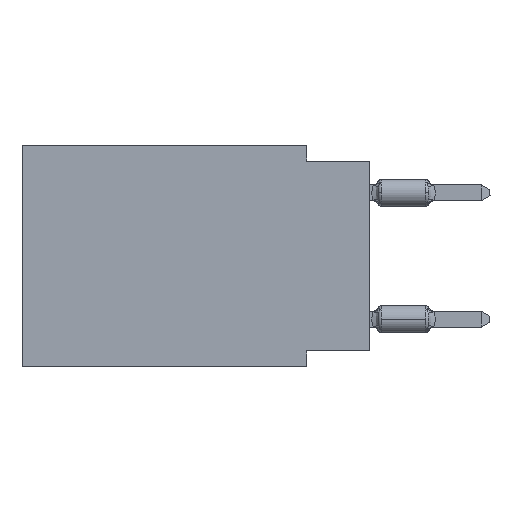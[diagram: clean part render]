
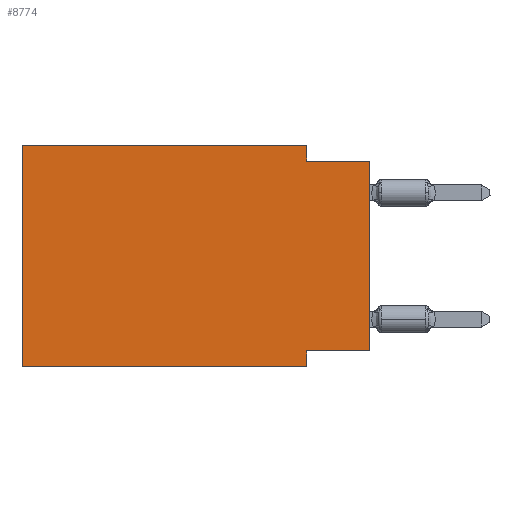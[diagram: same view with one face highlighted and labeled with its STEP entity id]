
A CAD part, left-side view. The second image highlights one B-rep face of the part: STEP entity #8774.
In plain terms, the highlighted planar face has unit normal (-1, 0, 0).
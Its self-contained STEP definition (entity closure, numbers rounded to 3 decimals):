
#552 = CARTESIAN_POINT ( 'NONE',  ( 0., 13.97, 0. ) ) ;
#872 = VECTOR ( 'NONE', #2977, 1000. ) ;
#1038 = ORIENTED_EDGE ( 'NONE', *, *, #6615, .T. ) ;
#1206 = CARTESIAN_POINT ( 'NONE',  ( 0., 2.54, -8.89 ) ) ;
#1652 = PLANE ( 'NONE',  #12553 ) ;
#1987 = ORIENTED_EDGE ( 'NONE', *, *, #8923, .F. ) ;
#2245 = CARTESIAN_POINT ( 'NONE',  ( 0., 2.54, -0.635 ) ) ;
#2977 = DIRECTION ( 'NONE',  ( 0., 0., -1. ) ) ;
#3429 = ORIENTED_EDGE ( 'NONE', *, *, #5360, .F. ) ;
#3430 = DIRECTION ( 'NONE',  ( 0., -1., 0. ) ) ;
#3570 = DIRECTION ( 'NONE',  ( 0., 0., -1. ) ) ;
#4036 = CARTESIAN_POINT ( 'NONE',  ( 0., 2.54, -8.255 ) ) ;
#4069 = CARTESIAN_POINT ( 'NONE',  ( 0., 2.54, 0. ) ) ;
#4144 = CARTESIAN_POINT ( 'NONE',  ( 0., 0., -8.255 ) ) ;
#4422 = VECTOR ( 'NONE', #27921, 1000. ) ;
#5103 = CARTESIAN_POINT ( 'NONE',  ( 0., 0., -0.635 ) ) ;
#5360 = EDGE_CURVE ( 'NONE', #18865, #16449, #18100, .T. ) ;
#5438 = CARTESIAN_POINT ( 'NONE',  ( 0., 2.54, 0. ) ) ;
#6615 = EDGE_CURVE ( 'NONE', #22072, #22114, #7286, .T. ) ;
#6619 = LINE ( 'NONE', #4144, #24721 ) ;
#6638 = EDGE_CURVE ( 'NONE', #8939, #22114, #17953, .T. ) ;
#7006 = DIRECTION ( 'NONE',  ( 0., -1., 0. ) ) ;
#7286 = LINE ( 'NONE', #16025, #12534 ) ;
#7339 = VECTOR ( 'NONE', #15163, 1000. ) ;
#7668 = LINE ( 'NONE', #12634, #13821 ) ;
#8774 = ADVANCED_FACE ( 'NONE', ( #25801 ), #1652, .F. ) ;
#8918 = ORIENTED_EDGE ( 'NONE', *, *, #18597, .F. ) ;
#8923 = EDGE_CURVE ( 'NONE', #22072, #18111, #6619, .T. ) ;
#8939 = VERTEX_POINT ( 'NONE', #2245 ) ;
#9040 = DIRECTION ( 'NONE',  ( 0., 0., 1. ) ) ;
#9163 = VERTEX_POINT ( 'NONE', #5438 ) ;
#9680 = VECTOR ( 'NONE', #18386, 1000. ) ;
#10164 = CARTESIAN_POINT ( 'NONE',  ( 0., 0., -0.635 ) ) ;
#10265 = CARTESIAN_POINT ( 'NONE',  ( 0., 2.54, -8.89 ) ) ;
#10452 = CARTESIAN_POINT ( 'NONE',  ( 0., 0., -8.255 ) ) ;
#11527 = CARTESIAN_POINT ( 'NONE',  ( 0., 13.97, 0. ) ) ;
#12534 = VECTOR ( 'NONE', #9040, 1000. ) ;
#12553 = AXIS2_PLACEMENT_3D ( 'NONE', #23609, #21689, #3570 ) ;
#12634 = CARTESIAN_POINT ( 'NONE',  ( 0., 13.97, 0. ) ) ;
#13142 = EDGE_CURVE ( 'NONE', #18865, #27840, #14449, .T. ) ;
#13821 = VECTOR ( 'NONE', #3430, 1000. ) ;
#14002 = ORIENTED_EDGE ( 'NONE', *, *, #16421, .F. ) ;
#14449 = LINE ( 'NONE', #26012, #4422 ) ;
#15028 = LINE ( 'NONE', #4069, #7339 ) ;
#15163 = DIRECTION ( 'NONE',  ( 0., 0., -1. ) ) ;
#15298 = EDGE_CURVE ( 'NONE', #16449, #9163, #7668, .T. ) ;
#15520 = DIRECTION ( 'NONE',  ( 0., 1., 0. ) ) ;
#16025 = CARTESIAN_POINT ( 'NONE',  ( 0., 0., 0. ) ) ;
#16421 = EDGE_CURVE ( 'NONE', #9163, #8939, #15028, .T. ) ;
#16449 = VERTEX_POINT ( 'NONE', #552 ) ;
#17813 = ORIENTED_EDGE ( 'NONE', *, *, #6638, .F. ) ;
#17953 = LINE ( 'NONE', #5103, #21885 ) ;
#18100 = LINE ( 'NONE', #11527, #9680 ) ;
#18111 = VERTEX_POINT ( 'NONE', #4036 ) ;
#18181 = EDGE_LOOP ( 'NONE', ( #1038, #17813, #14002, #20491, #3429, #22248, #8918, #1987 ) ) ;
#18386 = DIRECTION ( 'NONE',  ( 0., 0., 1. ) ) ;
#18597 = EDGE_CURVE ( 'NONE', #18111, #27840, #24785, .T. ) ;
#18865 = VERTEX_POINT ( 'NONE', #24751 ) ;
#20491 = ORIENTED_EDGE ( 'NONE', *, *, #15298, .F. ) ;
#21689 = DIRECTION ( 'NONE',  ( 1., 0., 0. ) ) ;
#21885 = VECTOR ( 'NONE', #7006, 1000. ) ;
#22072 = VERTEX_POINT ( 'NONE', #10452 ) ;
#22114 = VERTEX_POINT ( 'NONE', #10164 ) ;
#22248 = ORIENTED_EDGE ( 'NONE', *, *, #13142, .T. ) ;
#23609 = CARTESIAN_POINT ( 'NONE',  ( 0., 13.97, 0. ) ) ;
#24721 = VECTOR ( 'NONE', #15520, 1000. ) ;
#24751 = CARTESIAN_POINT ( 'NONE',  ( 0., 13.97, -8.89 ) ) ;
#24785 = LINE ( 'NONE', #1206, #872 ) ;
#25801 = FACE_OUTER_BOUND ( 'NONE', #18181, .T. ) ;
#26012 = CARTESIAN_POINT ( 'NONE',  ( 0., 13.97, -8.89 ) ) ;
#27840 = VERTEX_POINT ( 'NONE', #10265 ) ;
#27921 = DIRECTION ( 'NONE',  ( 0., -1., 0. ) ) ;
